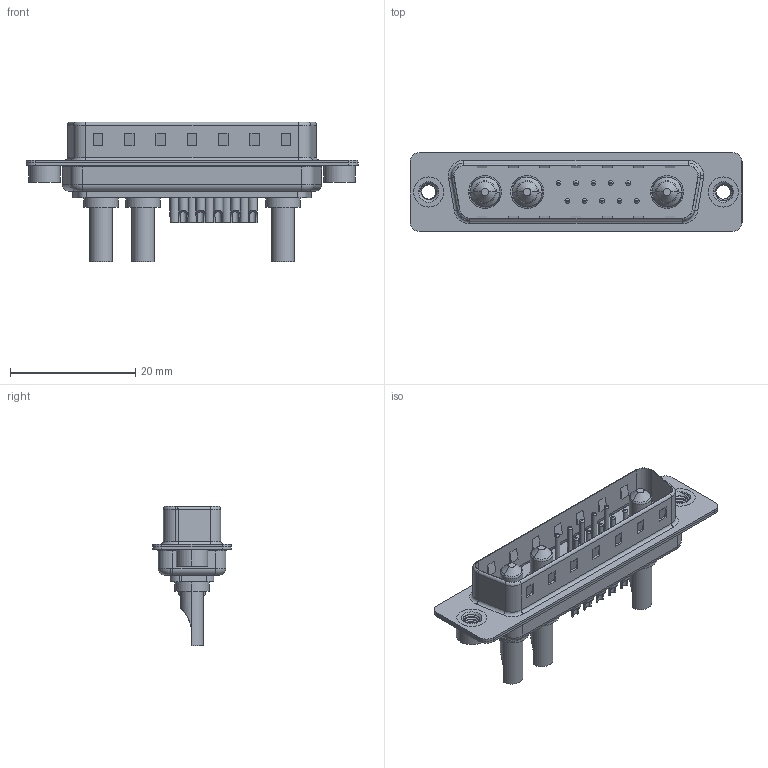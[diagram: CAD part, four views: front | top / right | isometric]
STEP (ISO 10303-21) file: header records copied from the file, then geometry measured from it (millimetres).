
FILE_DESCRIPTION (( 'STEP AP203' ), '1' );
FILE_NAME ('627-13W3222-2TA.STEP', '2019-05-26T12:01:42', ( '' ), ( '' ), 'SwSTEP 2.0', 'SolidWorks 2016', '' );
FILE_SCHEMA (( 'CONFIG_CONTROL_DESIGN' ));
Length unit declared in the file: millimetre
Products named in the file (9): 627Combo Threaded Rivet_A; Power Pin_20A SC; 627Combo Threaded Rivet_2; 627Combo Contact Row 1_22; 627Combo Contact Row 2_22; 627-13W3222-2TA; 627Combo Housing_13W3; 627Combo Shell Rear_25 Contacts; 627Combo Shell Front_25 Contacts
Assembly tree (18 placements, depth 2):
  627-13W3222-2TA
    627Combo Housing_13W3
    627Combo Shell Rear_25 Contacts
    627Combo Shell Front_25 Contacts
    627Combo Threaded Rivet_A
    Power Pin_20A SC  x3
    627Combo Threaded Rivet_2
    627Combo Contact Row 1_22  x5
    627Combo Contact Row 2_22  x5
Bounding box: 53 x 12.6 x 22.3 mm (x, y, z)
Volume: 2979.8 mm3; surface area: 7074.9 mm2
Topology: 21 solids, 21 shells, 883 faces, 2100 edges, 1293 vertices
Faces by surface type: cylinder 364, plane 300, torus 156, cone 51, bspline 12
Entity records: 21337 total; most frequent: CARTESIAN_POINT 6380, DIRECTION 3010, ORIENTED_EDGE 2768, EDGE_CURVE 1384, AXIS2_PLACEMENT_3D 1151, VERTEX_POINT 875, VECTOR 708, LINE 708
